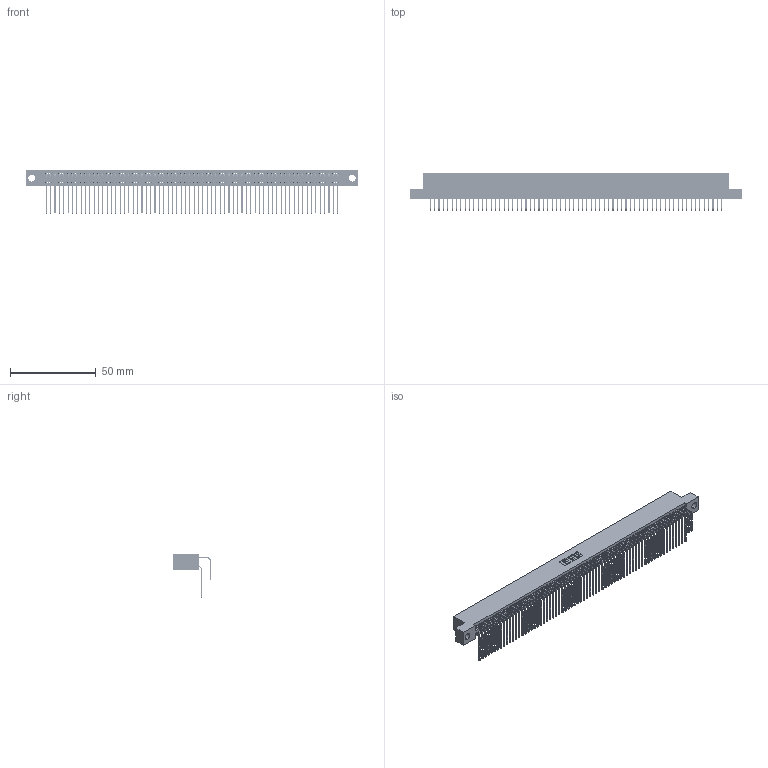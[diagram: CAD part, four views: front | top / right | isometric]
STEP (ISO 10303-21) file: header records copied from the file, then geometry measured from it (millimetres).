
FILE_DESCRIPTION (( 'STEP AP203' ), '1' );
FILE_NAME ('345-136-558-204.STEP', '2021-05-25T23:31:01', ( '' ), ( '' ), 'SwSTEP 2.0', 'SolidWorks 2020', '' );
FILE_SCHEMA (( 'CONFIG_CONTROL_DESIGN' ));
Length unit declared in the file: inch
Products named in the file (4): 345-136-558-204; 345-292-001_558 Tail - 2; 345-292-001_558 559 Tail - 1; 345 Part_Flush Mounting Lugs - 0.156 Dia-TI
Assembly tree (137 placements, depth 2):
  345-136-558-204
    345 Part_Flush Mounting Lugs - 0.156 Dia-TI
    345-292-001_558 559 Tail - 1  x68
    345-292-001_558 Tail - 2  x68
Bounding box: 193.93 x 21.83 x 25.53 mm (x, y, z)
Volume: 19758.4 mm3; surface area: 33250.6 mm2
Topology: 137 solids, 137 shells, 7212 faces, 21457 edges, 14122 vertices
Faces by surface type: plane 4854, cylinder 2358
Entity records: 51925 total; most frequent: CARTESIAN_POINT 8729, ORIENTED_EDGE 8610, DIRECTION 7637, EDGE_CURVE 4305, VECTOR 3861, LINE 3861, VERTEX_POINT 2866, AXIS2_PLACEMENT_3D 1888
